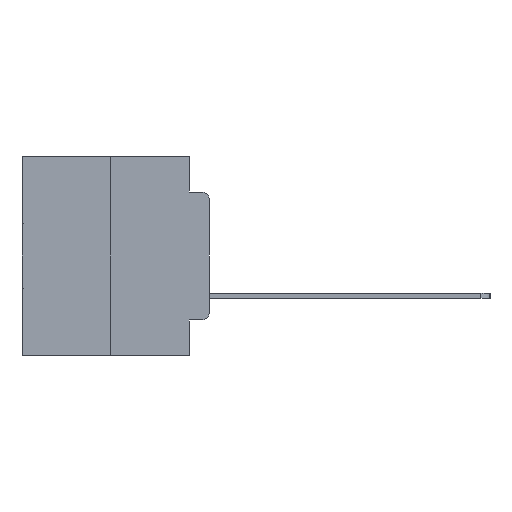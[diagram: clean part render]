
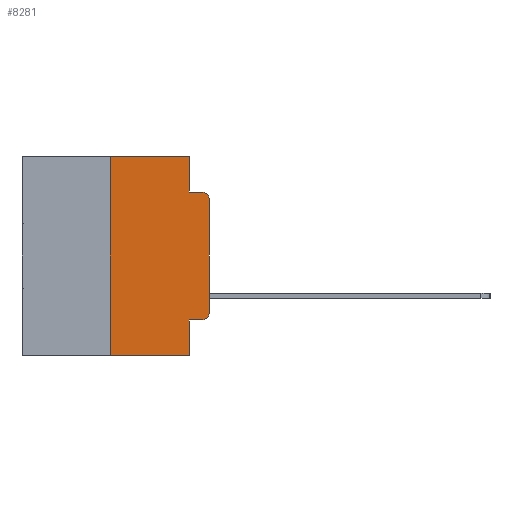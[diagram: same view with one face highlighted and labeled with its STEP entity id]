
A CAD part, left-side view. The second image highlights one B-rep face of the part: STEP entity #8281.
In plain terms, the highlighted planar face has unit normal (-1, 0, 0).
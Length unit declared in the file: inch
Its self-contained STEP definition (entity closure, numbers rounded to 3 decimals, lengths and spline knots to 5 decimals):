
#433 = VERTEX_POINT ( 'NONE', #21821 ) ;
#439 = DIRECTION ( 'NONE',  ( 0., -1., 0. ) ) ;
#577 = VERTEX_POINT ( 'NONE', #28571 ) ;
#951 = DIRECTION ( 'NONE',  ( 1., 0., 0. ) ) ;
#1460 = CARTESIAN_POINT ( 'NONE',  ( 0., 0.473, -0.5 ) ) ;
#1741 = CARTESIAN_POINT ( 'NONE',  ( 0., 0.25, 0. ) ) ;
#2223 = VECTOR ( 'NONE', #21279, 39.37008 ) ;
#2298 = ORIENTED_EDGE ( 'NONE', *, *, #20185, .F. ) ;
#3813 = LINE ( 'NONE', #20017, #20925 ) ;
#3925 = VERTEX_POINT ( 'NONE', #23723 ) ;
#4031 = DIRECTION ( 'NONE',  ( 0., -1., 0. ) ) ;
#4034 = VECTOR ( 'NONE', #4031, 39.37008 ) ;
#4328 = CARTESIAN_POINT ( 'NONE',  ( 0., 0.051, 0. ) ) ;
#4348 = VERTEX_POINT ( 'NONE', #25504 ) ;
#4551 = EDGE_CURVE ( 'NONE', #7020, #3925, #7874, .T. ) ;
#5723 = ORIENTED_EDGE ( 'NONE', *, *, #14068, .F. ) ;
#5724 = EDGE_CURVE ( 'NONE', #23081, #26663, #18234, .T. ) ;
#6874 = ORIENTED_EDGE ( 'NONE', *, *, #15940, .T. ) ;
#7020 = VERTEX_POINT ( 'NONE', #14986 ) ;
#7827 = CARTESIAN_POINT ( 'NONE',  ( 0., 0.051, 0. ) ) ;
#7874 = LINE ( 'NONE', #10997, #18699 ) ;
#8281 = ADVANCED_FACE ( 'NONE', ( #16148 ), #15308, .F. ) ;
#9320 = DIRECTION ( 'NONE',  ( -1., 0., 0. ) ) ;
#9604 = DIRECTION ( 'NONE',  ( -1., 0., 0. ) ) ;
#9900 = DIRECTION ( 'NONE',  ( 0., -1., 0. ) ) ;
#10707 = AXIS2_PLACEMENT_3D ( 'NONE', #22904, #9320, #25084 ) ;
#10997 = CARTESIAN_POINT ( 'NONE',  ( 0., 0., 0. ) ) ;
#11259 = CIRCLE ( 'NONE', #29325, 0.02 ) ;
#11392 = VECTOR ( 'NONE', #9900, 39.37008 ) ;
#11567 = EDGE_CURVE ( 'NONE', #4348, #577, #3813, .T. ) ;
#12379 = VERTEX_POINT ( 'NONE', #13551 ) ;
#12991 = CARTESIAN_POINT ( 'NONE',  ( 0., 0.473, 0. ) ) ;
#13051 = ORIENTED_EDGE ( 'NONE', *, *, #4551, .T. ) ;
#13551 = CARTESIAN_POINT ( 'NONE',  ( 0., 0.02, -0.0885 ) ) ;
#14068 = EDGE_CURVE ( 'NONE', #26663, #16480, #23946, .T. ) ;
#14258 = ORIENTED_EDGE ( 'NONE', *, *, #26554, .T. ) ;
#14656 = EDGE_CURVE ( 'NONE', #577, #7020, #11259, .T. ) ;
#14986 = CARTESIAN_POINT ( 'NONE',  ( 0., 0., -0.3915 ) ) ;
#15213 = EDGE_LOOP ( 'NONE', ( #13051, #6874, #18163, #5723, #24659, #2298, #14258, #26432, #24061, #22694 ) ) ;
#15216 = CARTESIAN_POINT ( 'NONE',  ( 0., 0.473, 0. ) ) ;
#15223 = DIRECTION ( 'NONE',  ( 0., 0., 1. ) ) ;
#15308 = PLANE ( 'NONE',  #18110 ) ;
#15637 = VECTOR ( 'NONE', #15223, 39.37008 ) ;
#15940 = EDGE_CURVE ( 'NONE', #3925, #12379, #29615, .T. ) ;
#16148 = FACE_OUTER_BOUND ( 'NONE', #15213, .T. ) ;
#16346 = LINE ( 'NONE', #19052, #2223 ) ;
#16480 = VERTEX_POINT ( 'NONE', #17894 ) ;
#17039 = DIRECTION ( 'NONE',  ( 0., 0., -1. ) ) ;
#17666 = DIRECTION ( 'NONE',  ( 0., 0., -1. ) ) ;
#17837 = DIRECTION ( 'NONE',  ( 0., 0., 1. ) ) ;
#17894 = CARTESIAN_POINT ( 'NONE',  ( 0., 0.051, -0.0885 ) ) ;
#18020 = LINE ( 'NONE', #1460, #4034 ) ;
#18110 = AXIS2_PLACEMENT_3D ( 'NONE', #15216, #951, #17666 ) ;
#18163 = ORIENTED_EDGE ( 'NONE', *, *, #26979, .F. ) ;
#18234 = LINE ( 'NONE', #12991, #11392 ) ;
#18699 = VECTOR ( 'NONE', #17837, 39.37008 ) ;
#19052 = CARTESIAN_POINT ( 'NONE',  ( 0., 0.051, 0. ) ) ;
#19337 = CARTESIAN_POINT ( 'NONE',  ( 0., 0.051, -0.0885 ) ) ;
#19488 = VECTOR ( 'NONE', #439, 39.37008 ) ;
#19647 = VERTEX_POINT ( 'NONE', #29057 ) ;
#20017 = CARTESIAN_POINT ( 'NONE',  ( 0., 0.051, -0.4115 ) ) ;
#20185 = EDGE_CURVE ( 'NONE', #19647, #23081, #28073, .T. ) ;
#20925 = VECTOR ( 'NONE', #22203, 39.37008 ) ;
#21279 = DIRECTION ( 'NONE',  ( 0., 0., -1. ) ) ;
#21821 = CARTESIAN_POINT ( 'NONE',  ( 0., 0.051, -0.5 ) ) ;
#22203 = DIRECTION ( 'NONE',  ( 0., -1., 0. ) ) ;
#22694 = ORIENTED_EDGE ( 'NONE', *, *, #14656, .T. ) ;
#22904 = CARTESIAN_POINT ( 'NONE',  ( 0., 0.02, -0.1085 ) ) ;
#23081 = VERTEX_POINT ( 'NONE', #1741 ) ;
#23157 = CARTESIAN_POINT ( 'NONE',  ( 0., 0.02, -0.3915 ) ) ;
#23259 = VECTOR ( 'NONE', #17039, 39.37008 ) ;
#23723 = CARTESIAN_POINT ( 'NONE',  ( 0., 0., -0.1085 ) ) ;
#23946 = LINE ( 'NONE', #7827, #23259 ) ;
#24000 = EDGE_CURVE ( 'NONE', #4348, #433, #16346, .T. ) ;
#24061 = ORIENTED_EDGE ( 'NONE', *, *, #11567, .T. ) ;
#24094 = CARTESIAN_POINT ( 'NONE',  ( 0., 0.25, 0. ) ) ;
#24659 = ORIENTED_EDGE ( 'NONE', *, *, #5724, .F. ) ;
#25084 = DIRECTION ( 'NONE',  ( 0., 0., -1. ) ) ;
#25277 = LINE ( 'NONE', #19337, #19488 ) ;
#25340 = DIRECTION ( 'NONE',  ( 0., 0., -1. ) ) ;
#25504 = CARTESIAN_POINT ( 'NONE',  ( 0., 0.051, -0.4115 ) ) ;
#26432 = ORIENTED_EDGE ( 'NONE', *, *, #24000, .F. ) ;
#26554 = EDGE_CURVE ( 'NONE', #19647, #433, #18020, .T. ) ;
#26663 = VERTEX_POINT ( 'NONE', #4328 ) ;
#26979 = EDGE_CURVE ( 'NONE', #16480, #12379, #25277, .T. ) ;
#28073 = LINE ( 'NONE', #24094, #15637 ) ;
#28571 = CARTESIAN_POINT ( 'NONE',  ( 0., 0.02, -0.4115 ) ) ;
#29057 = CARTESIAN_POINT ( 'NONE',  ( 0., 0.25, -0.5 ) ) ;
#29325 = AXIS2_PLACEMENT_3D ( 'NONE', #23157, #9604, #25340 ) ;
#29615 = CIRCLE ( 'NONE', #10707, 0.02 ) ;
